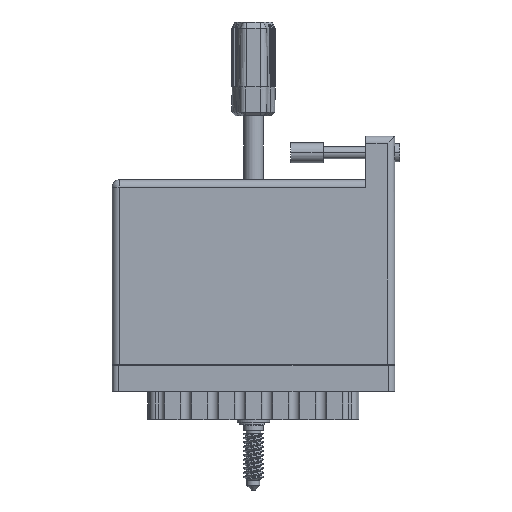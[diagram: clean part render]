
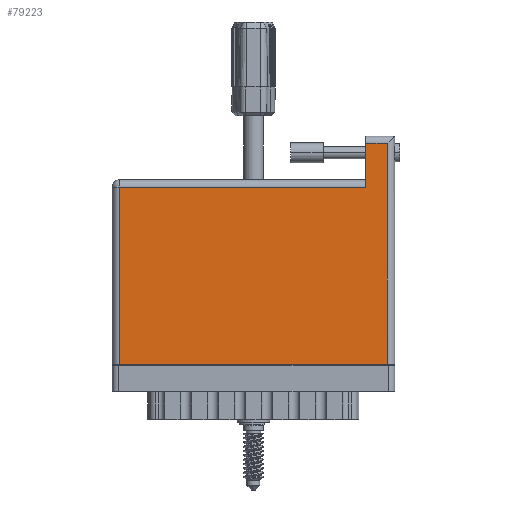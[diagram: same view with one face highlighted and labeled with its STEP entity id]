
A CAD part, front view. The second image highlights one B-rep face of the part: STEP entity #79223.
In plain terms, the highlighted face is planar.
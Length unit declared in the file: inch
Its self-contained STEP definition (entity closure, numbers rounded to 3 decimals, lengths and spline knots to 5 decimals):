
#825 = LINE ( 'NONE', #50323, #1884 ) ;
#1884 = VECTOR ( 'NONE', #82473, 39.37008 ) ;
#3175 = LINE ( 'NONE', #18896, #38573 ) ;
#3391 = VERTEX_POINT ( 'NONE', #61045 ) ;
#4664 = DIRECTION ( 'NONE',  ( 1., 0., 0. ) ) ;
#5186 = VECTOR ( 'NONE', #4664, 39.37008 ) ;
#8852 = ORIENTED_EDGE ( 'NONE', *, *, #61798, .T. ) ;
#11594 = CARTESIAN_POINT ( 'NONE',  ( 2.438, 2.125, 0. ) ) ;
#12933 = ORIENTED_EDGE ( 'NONE', *, *, #23165, .T. ) ;
#17221 = CARTESIAN_POINT ( 'NONE',  ( 2.648, 2.195, 0. ) ) ;
#18896 = CARTESIAN_POINT ( 'NONE',  ( 0., 2.125, 0. ) ) ;
#20262 = LINE ( 'NONE', #79763, #52638 ) ;
#22979 = CARTESIAN_POINT ( 'NONE',  ( 0., 1.775, 0. ) ) ;
#23165 = EDGE_CURVE ( 'NONE', #76819, #81663, #39467, .T. ) ;
#24286 = DIRECTION ( 'NONE',  ( 0., 1., 0. ) ) ;
#24548 = EDGE_CURVE ( 'NONE', #46977, #76819, #825, .T. ) ;
#26497 = FACE_OUTER_BOUND ( 'NONE', #48654, .T. ) ;
#30762 = EDGE_CURVE ( 'NONE', #49748, #45896, #3175, .T. ) ;
#35492 = ORIENTED_EDGE ( 'NONE', *, *, #41187, .T. ) ;
#36825 = PLANE ( 'NONE',  #46697 ) ;
#38573 = VECTOR ( 'NONE', #43780, 39.37008 ) ;
#39467 = LINE ( 'NONE', #74111, #54653 ) ;
#41187 = EDGE_CURVE ( 'NONE', #45896, #46977, #20262, .T. ) ;
#41586 = DIRECTION ( 'NONE',  ( 0., -1., 0. ) ) ;
#41910 = EDGE_CURVE ( 'NONE', #3391, #49748, #45406, .T. ) ;
#43780 = DIRECTION ( 'NONE',  ( -1., 0., 0. ) ) ;
#45320 = CARTESIAN_POINT ( 'NONE',  ( 2.438, 1.705, 0. ) ) ;
#45406 = LINE ( 'NONE', #17221, #64634 ) ;
#45896 = VERTEX_POINT ( 'NONE', #11594 ) ;
#46697 = AXIS2_PLACEMENT_3D ( 'NONE', #22979, #55760, #68504 ) ;
#46977 = VERTEX_POINT ( 'NONE', #45320 ) ;
#47384 = CARTESIAN_POINT ( 'NONE',  ( 0.07, 1.705, 0. ) ) ;
#48654 = EDGE_LOOP ( 'NONE', ( #67868, #12933, #8852, #74895, #58864, #35492 ) ) ;
#49748 = VERTEX_POINT ( 'NONE', #56374 ) ;
#50323 = CARTESIAN_POINT ( 'NONE',  ( 0., 1.705, 0. ) ) ;
#52638 = VECTOR ( 'NONE', #73042, 39.37008 ) ;
#54653 = VECTOR ( 'NONE', #41586, 39.37008 ) ;
#55760 = DIRECTION ( 'NONE',  ( 0., 0., -1. ) ) ;
#56371 = CARTESIAN_POINT ( 'NONE',  ( 0., 0., 0. ) ) ;
#56374 = CARTESIAN_POINT ( 'NONE',  ( 2.648, 2.125, 0. ) ) ;
#58864 = ORIENTED_EDGE ( 'NONE', *, *, #30762, .T. ) ;
#61045 = CARTESIAN_POINT ( 'NONE',  ( 2.648, 0., 0. ) ) ;
#61798 = EDGE_CURVE ( 'NONE', #81663, #3391, #70924, .T. ) ;
#64634 = VECTOR ( 'NONE', #24286, 39.37008 ) ;
#67868 = ORIENTED_EDGE ( 'NONE', *, *, #24548, .T. ) ;
#68504 = DIRECTION ( 'NONE',  ( -1., 0., 0. ) ) ;
#70924 = LINE ( 'NONE', #56371, #5186 ) ;
#73042 = DIRECTION ( 'NONE',  ( 0., -1., 0. ) ) ;
#74111 = CARTESIAN_POINT ( 'NONE',  ( 0.07, 0., 0. ) ) ;
#74895 = ORIENTED_EDGE ( 'NONE', *, *, #41910, .T. ) ;
#75148 = CARTESIAN_POINT ( 'NONE',  ( 0.07, 0., 0. ) ) ;
#76819 = VERTEX_POINT ( 'NONE', #47384 ) ;
#79223 = ADVANCED_FACE ( 'NONE', ( #26497 ), #36825, .F. ) ;
#79763 = CARTESIAN_POINT ( 'NONE',  ( 2.438, 2.195, 0. ) ) ;
#81663 = VERTEX_POINT ( 'NONE', #75148 ) ;
#82473 = DIRECTION ( 'NONE',  ( -1., 0., 0. ) ) ;
